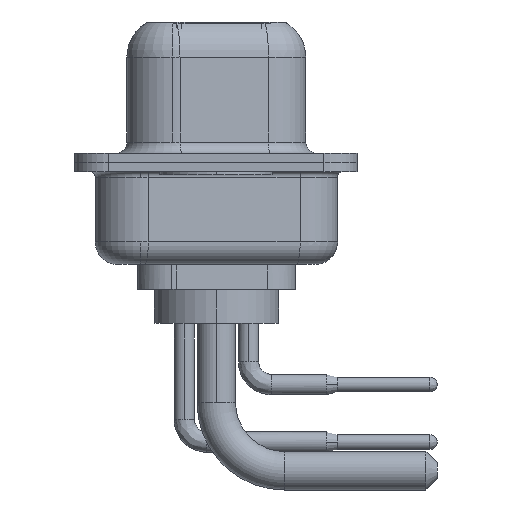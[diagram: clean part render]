
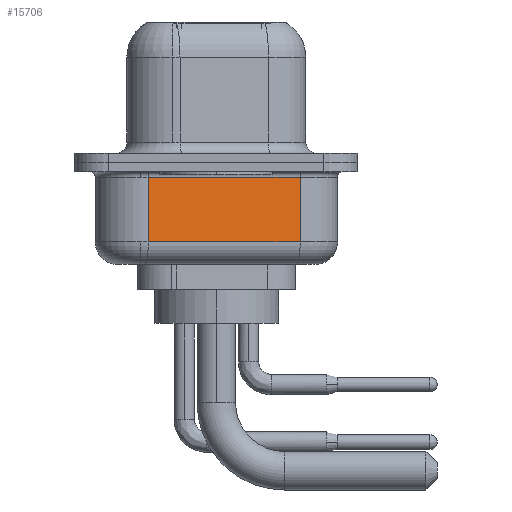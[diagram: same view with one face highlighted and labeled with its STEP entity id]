
A CAD part, left-side view. The second image highlights one B-rep face of the part: STEP entity #15706.
In plain terms, the highlighted planar face has unit normal (-0.985, -0.174, 0).
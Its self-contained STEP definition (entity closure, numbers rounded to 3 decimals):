
#43 = VECTOR ( 'NONE', #7515, 1000. ) ;
#547 = VERTEX_POINT ( 'NONE', #13781 ) ;
#2955 = PLANE ( 'NONE',  #13891 ) ;
#3089 = ORIENTED_EDGE ( 'NONE', *, *, #14924, .T. ) ;
#4484 = CARTESIAN_POINT ( 'NONE',  ( 2.88, 3.003, -4.5 ) ) ;
#6356 = DIRECTION ( 'NONE',  ( -0.174, 0.985, 0. ) ) ;
#7515 = DIRECTION ( 'NONE',  ( 0.174, -0.985, 0. ) ) ;
#7605 = CARTESIAN_POINT ( 'NONE',  ( 4.062, -3.697, -4.5 ) ) ;
#8761 = CARTESIAN_POINT ( 'NONE',  ( 2.88, 3.003, -0.65 ) ) ;
#11114 = VERTEX_POINT ( 'NONE', #8761 ) ;
#11358 = FACE_OUTER_BOUND ( 'NONE', #17910, .T. ) ;
#11540 = DIRECTION ( 'NONE',  ( 0., 0., 1. ) ) ;
#11882 = CARTESIAN_POINT ( 'NONE',  ( 2.88, 3.003, -4.5 ) ) ;
#12933 = EDGE_CURVE ( 'NONE', #14452, #17901, #22980, .T. ) ;
#13185 = LINE ( 'NONE', #7605, #14592 ) ;
#13268 = ORIENTED_EDGE ( 'NONE', *, *, #19586, .F. ) ;
#13684 = LINE ( 'NONE', #20759, #22741 ) ;
#13781 = CARTESIAN_POINT ( 'NONE',  ( 4.062, -3.697, -0.65 ) ) ;
#13891 = AXIS2_PLACEMENT_3D ( 'NONE', #4484, #18451, #16944 ) ;
#14452 = VERTEX_POINT ( 'NONE', #15190 ) ;
#14592 = VECTOR ( 'NONE', #14699, 1000. ) ;
#14699 = DIRECTION ( 'NONE',  ( 0., 0., 1. ) ) ;
#14924 = EDGE_CURVE ( 'NONE', #17901, #547, #13185, .T. ) ;
#15190 = CARTESIAN_POINT ( 'NONE',  ( 2.88, 3.003, -3.5 ) ) ;
#15706 = ADVANCED_FACE ( 'NONE', ( #11358 ), #2955, .F. ) ;
#16944 = DIRECTION ( 'NONE',  ( -0.174, 0.985, 0. ) ) ;
#17901 = VERTEX_POINT ( 'NONE', #19107 ) ;
#17910 = EDGE_LOOP ( 'NONE', ( #13268, #21703, #3089, #21834 ) ) ;
#18215 = CARTESIAN_POINT ( 'NONE',  ( 2.88, 3.003, -3.5 ) ) ;
#18451 = DIRECTION ( 'NONE',  ( 0.985, 0.174, 0. ) ) ;
#18640 = EDGE_CURVE ( 'NONE', #547, #11114, #13684, .T. ) ;
#19107 = CARTESIAN_POINT ( 'NONE',  ( 4.062, -3.697, -3.5 ) ) ;
#19586 = EDGE_CURVE ( 'NONE', #14452, #11114, #20367, .T. ) ;
#19746 = VECTOR ( 'NONE', #11540, 1000. ) ;
#20367 = LINE ( 'NONE', #11882, #19746 ) ;
#20759 = CARTESIAN_POINT ( 'NONE',  ( 2.88, 3.003, -0.65 ) ) ;
#21703 = ORIENTED_EDGE ( 'NONE', *, *, #12933, .T. ) ;
#21834 = ORIENTED_EDGE ( 'NONE', *, *, #18640, .T. ) ;
#22741 = VECTOR ( 'NONE', #6356, 1000. ) ;
#22980 = LINE ( 'NONE', #18215, #43 ) ;
